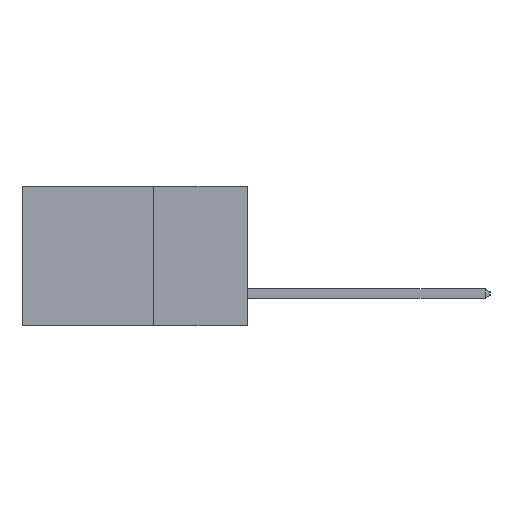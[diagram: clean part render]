
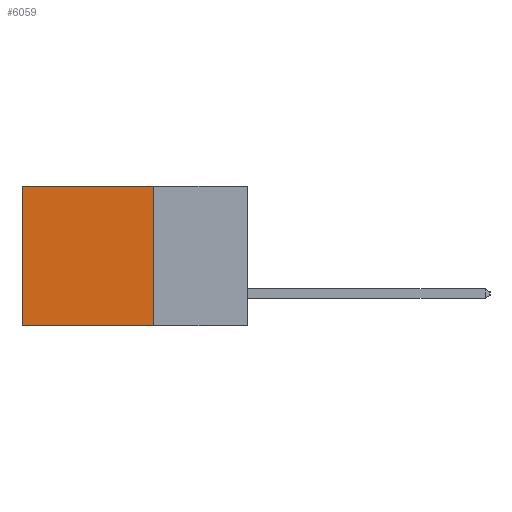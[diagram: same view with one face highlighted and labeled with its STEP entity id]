
A CAD part, left-side view. The second image highlights one B-rep face of the part: STEP entity #6059.
In plain terms, the highlighted planar face has unit normal (-1, 0, 0).
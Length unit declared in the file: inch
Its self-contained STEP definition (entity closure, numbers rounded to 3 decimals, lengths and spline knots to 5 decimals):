
#29 = ORIENTED_EDGE ( 'NONE', *, *, #13806, .T. ) ;
#116 = LINE ( 'NONE', #24399, #11593 ) ;
#1515 = LINE ( 'NONE', #3221, #27128 ) ;
#1685 = VERTEX_POINT ( 'NONE', #25442 ) ;
#1779 = EDGE_CURVE ( 'NONE', #6085, #8125, #14904, .T. ) ;
#2049 = ORIENTED_EDGE ( 'NONE', *, *, #12047, .F. ) ;
#3221 = CARTESIAN_POINT ( 'NONE',  ( 0.298, 0.25, 0. ) ) ;
#4312 = DIRECTION ( 'NONE',  ( 0., 0., -1. ) ) ;
#6059 = ADVANCED_FACE ( 'NONE', ( #18216 ), #12692, .F. ) ;
#6085 = VERTEX_POINT ( 'NONE', #8268 ) ;
#7653 = EDGE_LOOP ( 'NONE', ( #15003, #22269, #2049, #29 ) ) ;
#8125 = VERTEX_POINT ( 'NONE', #11170 ) ;
#8246 = EDGE_CURVE ( 'NONE', #22448, #8125, #116, .T. ) ;
#8268 = CARTESIAN_POINT ( 'NONE',  ( 0.298, 0.6, 0. ) ) ;
#9227 = VECTOR ( 'NONE', #25745, 39.37008 ) ;
#10687 = CARTESIAN_POINT ( 'NONE',  ( 0.298, 0.25, -0.37 ) ) ;
#10975 = AXIS2_PLACEMENT_3D ( 'NONE', #19669, #14130, #4312 ) ;
#11170 = CARTESIAN_POINT ( 'NONE',  ( 0.298, 0.6, -0.37 ) ) ;
#11593 = VECTOR ( 'NONE', #11722, 39.37008 ) ;
#11722 = DIRECTION ( 'NONE',  ( 0., 1., 0. ) ) ;
#12047 = EDGE_CURVE ( 'NONE', #1685, #22448, #24947, .T. ) ;
#12692 = PLANE ( 'NONE',  #10975 ) ;
#13806 = EDGE_CURVE ( 'NONE', #1685, #6085, #1515, .T. ) ;
#14130 = DIRECTION ( 'NONE',  ( 1., 0., 0. ) ) ;
#14904 = LINE ( 'NONE', #21646, #9227 ) ;
#15003 = ORIENTED_EDGE ( 'NONE', *, *, #1779, .T. ) ;
#15007 = CARTESIAN_POINT ( 'NONE',  ( 0.298, 0.25, 0. ) ) ;
#18216 = FACE_OUTER_BOUND ( 'NONE', #7653, .T. ) ;
#19669 = CARTESIAN_POINT ( 'NONE',  ( 0.298, 0.25, 0. ) ) ;
#21646 = CARTESIAN_POINT ( 'NONE',  ( 0.298, 0.6, 0. ) ) ;
#22269 = ORIENTED_EDGE ( 'NONE', *, *, #8246, .F. ) ;
#22441 = DIRECTION ( 'NONE',  ( 0., 1., 0. ) ) ;
#22448 = VERTEX_POINT ( 'NONE', #10687 ) ;
#24304 = VECTOR ( 'NONE', #25564, 39.37008 ) ;
#24399 = CARTESIAN_POINT ( 'NONE',  ( 0.298, 0.25, -0.37 ) ) ;
#24947 = LINE ( 'NONE', #15007, #24304 ) ;
#25442 = CARTESIAN_POINT ( 'NONE',  ( 0.298, 0.25, 0. ) ) ;
#25564 = DIRECTION ( 'NONE',  ( 0., 0., -1. ) ) ;
#25745 = DIRECTION ( 'NONE',  ( 0., 0., -1. ) ) ;
#27128 = VECTOR ( 'NONE', #22441, 39.37008 ) ;
